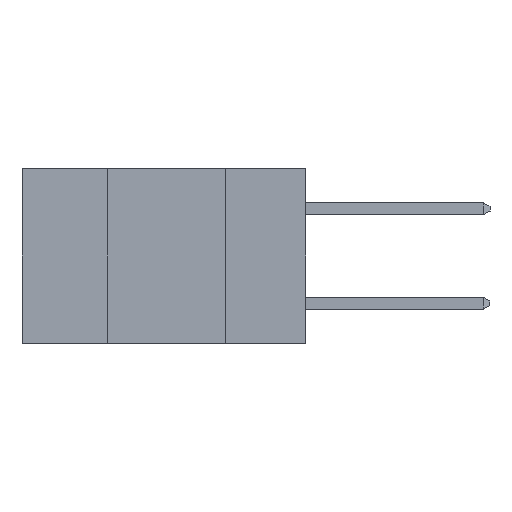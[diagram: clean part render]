
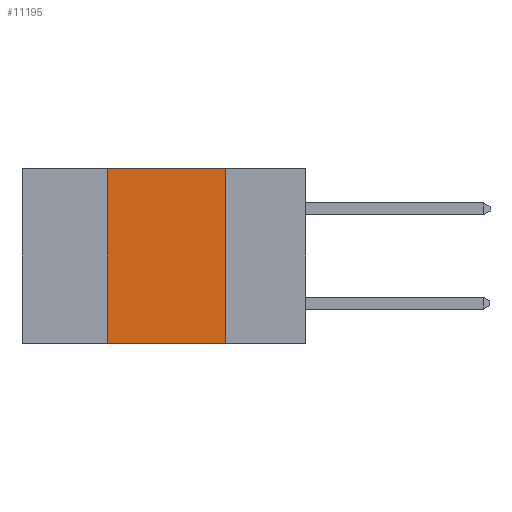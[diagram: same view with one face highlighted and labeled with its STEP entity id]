
A CAD part, left-side view. The second image highlights one B-rep face of the part: STEP entity #11195.
In plain terms, the highlighted planar face has unit normal (-1, 0, 0).
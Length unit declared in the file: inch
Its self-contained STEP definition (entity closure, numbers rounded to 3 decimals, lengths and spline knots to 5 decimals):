
#1329 = CARTESIAN_POINT ( 'NONE',  ( 0., 0.6, 0. ) ) ;
#1745 = LINE ( 'NONE', #1329, #12337 ) ;
#2150 = CARTESIAN_POINT ( 'NONE',  ( 0., 0.6, 0. ) ) ;
#2433 = FACE_OUTER_BOUND ( 'NONE', #10136, .T. ) ;
#2539 = CARTESIAN_POINT ( 'NONE',  ( 0., 0.17, 0. ) ) ;
#3021 = VERTEX_POINT ( 'NONE', #11425 ) ;
#3153 = VECTOR ( 'NONE', #11451, 39.37008 ) ;
#3435 = AXIS2_PLACEMENT_3D ( 'NONE', #2150, #7781, #7547 ) ;
#3562 = DIRECTION ( 'NONE',  ( 0., -1., 0. ) ) ;
#5130 = VERTEX_POINT ( 'NONE', #10392 ) ;
#5729 = LINE ( 'NONE', #2539, #8186 ) ;
#5942 = LINE ( 'NONE', #8505, #3153 ) ;
#6510 = PLANE ( 'NONE',  #3435 ) ;
#7368 = ORIENTED_EDGE ( 'NONE', *, *, #11845, .F. ) ;
#7445 = ORIENTED_EDGE ( 'NONE', *, *, #10708, .F. ) ;
#7547 = DIRECTION ( 'NONE',  ( 0., 0., -1. ) ) ;
#7615 = ORIENTED_EDGE ( 'NONE', *, *, #11224, .F. ) ;
#7627 = ORIENTED_EDGE ( 'NONE', *, *, #10545, .T. ) ;
#7716 = VECTOR ( 'NONE', #12459, 39.37008 ) ;
#7781 = DIRECTION ( 'NONE',  ( 1., 0., 0. ) ) ;
#8117 = CARTESIAN_POINT ( 'NONE',  ( 0., 0.42, 0. ) ) ;
#8186 = VECTOR ( 'NONE', #8802, 39.37008 ) ;
#8207 = VERTEX_POINT ( 'NONE', #8117 ) ;
#8505 = CARTESIAN_POINT ( 'NONE',  ( 0., 0.6, -0.37 ) ) ;
#8518 = CARTESIAN_POINT ( 'NONE',  ( 0., 0.17, -0.37 ) ) ;
#8802 = DIRECTION ( 'NONE',  ( 0., 0., -1. ) ) ;
#10136 = EDGE_LOOP ( 'NONE', ( #7368, #7445, #7615, #7627 ) ) ;
#10339 = LINE ( 'NONE', #11480, #7716 ) ;
#10392 = CARTESIAN_POINT ( 'NONE',  ( 0., 0.42, -0.37 ) ) ;
#10545 = EDGE_CURVE ( 'NONE', #5130, #11799, #5942, .T. ) ;
#10708 = EDGE_CURVE ( 'NONE', #8207, #3021, #1745, .T. ) ;
#11195 = ADVANCED_FACE ( 'NONE', ( #2433 ), #6510, .F. ) ;
#11224 = EDGE_CURVE ( 'NONE', #5130, #8207, #10339, .T. ) ;
#11425 = CARTESIAN_POINT ( 'NONE',  ( 0., 0.17, 0. ) ) ;
#11451 = DIRECTION ( 'NONE',  ( 0., -1., 0. ) ) ;
#11480 = CARTESIAN_POINT ( 'NONE',  ( 0., 0.42, 0. ) ) ;
#11799 = VERTEX_POINT ( 'NONE', #8518 ) ;
#11845 = EDGE_CURVE ( 'NONE', #3021, #11799, #5729, .T. ) ;
#12337 = VECTOR ( 'NONE', #3562, 39.37008 ) ;
#12459 = DIRECTION ( 'NONE',  ( 0., 0., 1. ) ) ;
